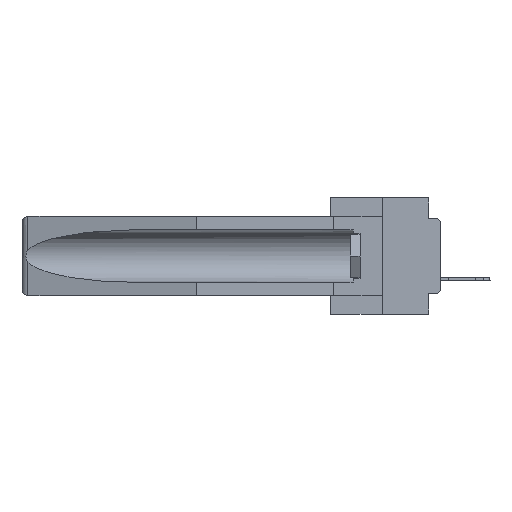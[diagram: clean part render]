
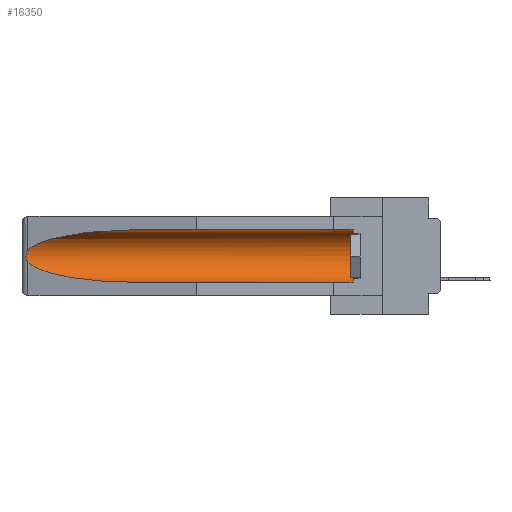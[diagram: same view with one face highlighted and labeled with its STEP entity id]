
A CAD part, left-side view. The second image highlights one B-rep face of the part: STEP entity #16350.
In plain terms, the highlighted cylindrical face has radius 2.857 mm (diameter 5.715 mm), a partial arc.
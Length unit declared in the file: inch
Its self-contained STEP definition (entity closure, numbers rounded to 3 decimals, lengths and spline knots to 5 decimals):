
#13 = CARTESIAN_POINT ( 'NONE',  ( 0.26537, 1.52718, -0.14972 ) ) ;
#753 = EDGE_CURVE ( 'NONE', #4381, #26947, #6992, .T. ) ;
#2082 = CARTESIAN_POINT ( 'NONE',  ( 0.155, 0.126, -0.059 ) ) ;
#2334 = ORIENTED_EDGE ( 'NONE', *, *, #6792, .T. ) ;
#2354 = CARTESIAN_POINT ( 'NONE',  ( 0.155, 1.07973, -0.059 ) ) ;
#2435 = CARTESIAN_POINT ( 'NONE',  ( 0.155, 1.07973, -0.284 ) ) ;
#3371 = AXIS2_PLACEMENT_3D ( 'NONE', #24261, #18692, #26468 ) ;
#3381 = CARTESIAN_POINT ( 'NONE',  ( 0.2673, 1.53269, -0.17917 ) ) ;
#4381 = VERTEX_POINT ( 'NONE', #2082 ) ;
#4632 = ORIENTED_EDGE ( 'NONE', *, *, #15241, .T. ) ;
#6214 = CARTESIAN_POINT ( 'NONE',  ( 0.2675, 1.53308, -0.16763 ) ) ;
#6224 = CARTESIAN_POINT ( 'NONE',  ( 0.155, 0.126, -0.284 ) ) ;
#6792 = EDGE_CURVE ( 'NONE', #25559, #4381, #17921, .T. ) ;
#6992 = LINE ( 'NONE', #16790, #33036 ) ;
#8534 = B_SPLINE_CURVE_WITH_KNOTS ( 'NONE', 3,
 ( #26836, #21597, #31891, #8598, #6214, #16520, #3381, #13690, #24297, #14020 ),
 .UNSPECIFIED., .F., .F.,
 ( 4, 2, 2, 2, 4 ),
 ( 0., 0.00029, 0.00058, 0.00087, 0.00117 ),
 .UNSPECIFIED. ) ;
#8598 = CARTESIAN_POINT ( 'NONE',  ( 0.2673, 1.5327, -0.16383 ) ) ;
#8639 = CARTESIAN_POINT ( 'NONE',  ( 0.155, -0.30754, -0.1715 ) ) ;
#8984 = CYLINDRICAL_SURFACE ( 'NONE', #32797, 0.1125 ) ;
#9365 = DIRECTION ( 'NONE',  ( 0., 1., 0. ) ) ;
#10336 = CARTESIAN_POINT ( 'NONE',  ( 0.26537, 1.52718, -0.14972 ) ) ;
#10584 = EDGE_CURVE ( 'NONE', #25559, #24797, #32493, .T. ) ;
#11693 = DIRECTION ( 'NONE',  ( 0., 1., 0. ) ) ;
#12263 = VERTEX_POINT ( 'NONE', #13 ) ;
#13038 = CARTESIAN_POINT ( 'NONE',  ( 0.21114, 1.30732, -0.059 ) ) ;
#13690 = CARTESIAN_POINT ( 'NONE',  ( 0.26655, 1.53094, -0.18657 ) ) ;
#14020 = CARTESIAN_POINT ( 'NONE',  ( 0.26537, 1.52718, -0.19328 ) ) ;
#14051 =( BOUNDED_CURVE ( )  B_SPLINE_CURVE ( 3, ( #22946, #33250, #25801, #28495 ),
 .UNSPECIFIED., .F., .F. ) 
 B_SPLINE_CURVE_WITH_KNOTS ( ( 4, 4 ),
 ( 0.1948, 1.5708 ),
 .UNSPECIFIED. ) 
 CURVE ( )  GEOMETRIC_REPRESENTATION_ITEM ( )  RATIONAL_B_SPLINE_CURVE ( ( 1., 0.848, 0.848, 1. ) ) 
 REPRESENTATION_ITEM ( '' )  );
#14454 = DIRECTION ( 'NONE',  ( 0., 1., 0. ) ) ;
#15241 = EDGE_CURVE ( 'NONE', #23322, #24797, #14051, .T. ) ;
#16350 = ADVANCED_FACE ( 'NONE', ( #19605 ), #8984, .F. ) ;
#16520 = CARTESIAN_POINT ( 'NONE',  ( 0.2675, 1.53308, -0.17534 ) ) ;
#16790 = CARTESIAN_POINT ( 'NONE',  ( 0.155, -0.30754, -0.059 ) ) ;
#16804 = ORIENTED_EDGE ( 'NONE', *, *, #10584, .F. ) ;
#17299 = EDGE_CURVE ( 'NONE', #26947, #12263, #29125, .T. ) ;
#17921 = CIRCLE ( 'NONE', #3371, 0.1125 ) ;
#18692 = DIRECTION ( 'NONE',  ( 0., -1., 0. ) ) ;
#19605 = FACE_OUTER_BOUND ( 'NONE', #25569, .T. ) ;
#21597 = CARTESIAN_POINT ( 'NONE',  ( 0.26597, 1.52961, -0.15275 ) ) ;
#22946 = CARTESIAN_POINT ( 'NONE',  ( 0.26537, 1.52718, -0.19328 ) ) ;
#23319 = CARTESIAN_POINT ( 'NONE',  ( 0.155, 1.07973, -0.059 ) ) ;
#23322 = VERTEX_POINT ( 'NONE', #26586 ) ;
#23808 = ORIENTED_EDGE ( 'NONE', *, *, #17299, .T. ) ;
#24261 = CARTESIAN_POINT ( 'NONE',  ( 0.155, 0.126, -0.1715 ) ) ;
#24297 = CARTESIAN_POINT ( 'NONE',  ( 0.26597, 1.5296, -0.19026 ) ) ;
#24797 = VERTEX_POINT ( 'NONE', #2435 ) ;
#25559 = VERTEX_POINT ( 'NONE', #6224 ) ;
#25569 = EDGE_LOOP ( 'NONE', ( #23808, #31619, #4632, #16804, #2334, #26772 ) ) ;
#25801 = CARTESIAN_POINT ( 'NONE',  ( 0.21114, 1.30732, -0.284 ) ) ;
#26157 = VECTOR ( 'NONE', #9365, 39.37008 ) ;
#26468 = DIRECTION ( 'NONE',  ( 0., 0., 1. ) ) ;
#26586 = CARTESIAN_POINT ( 'NONE',  ( 0.26537, 1.52718, -0.19328 ) ) ;
#26772 = ORIENTED_EDGE ( 'NONE', *, *, #753, .T. ) ;
#26836 = CARTESIAN_POINT ( 'NONE',  ( 0.26537, 1.52718, -0.14972 ) ) ;
#26888 = DIRECTION ( 'NONE',  ( 0., 0., 1. ) ) ;
#26927 = CARTESIAN_POINT ( 'NONE',  ( 0.155, -0.30754, -0.284 ) ) ;
#26947 = VERTEX_POINT ( 'NONE', #2354 ) ;
#28379 = CARTESIAN_POINT ( 'NONE',  ( 0.25451, 1.48313, -0.09465 ) ) ;
#28495 = CARTESIAN_POINT ( 'NONE',  ( 0.155, 1.07973, -0.284 ) ) ;
#29125 =( BOUNDED_CURVE ( )  B_SPLINE_CURVE ( 3, ( #23319, #13038, #28379, #10336 ),
 .UNSPECIFIED., .F., .F. ) 
 B_SPLINE_CURVE_WITH_KNOTS ( ( 4, 4 ),
 ( 4.71239, 6.08839 ),
 .UNSPECIFIED. ) 
 CURVE ( )  GEOMETRIC_REPRESENTATION_ITEM ( )  RATIONAL_B_SPLINE_CURVE ( ( 1., 0.848, 0.848, 1. ) ) 
 REPRESENTATION_ITEM ( '' )  );
#30600 = EDGE_CURVE ( 'NONE', #12263, #23322, #8534, .T. ) ;
#31619 = ORIENTED_EDGE ( 'NONE', *, *, #30600, .T. ) ;
#31891 = CARTESIAN_POINT ( 'NONE',  ( 0.26654, 1.53092, -0.15636 ) ) ;
#32493 = LINE ( 'NONE', #26927, #26157 ) ;
#32797 = AXIS2_PLACEMENT_3D ( 'NONE', #8639, #11693, #26888 ) ;
#33036 = VECTOR ( 'NONE', #14454, 39.37008 ) ;
#33250 = CARTESIAN_POINT ( 'NONE',  ( 0.25451, 1.48313, -0.24835 ) ) ;
